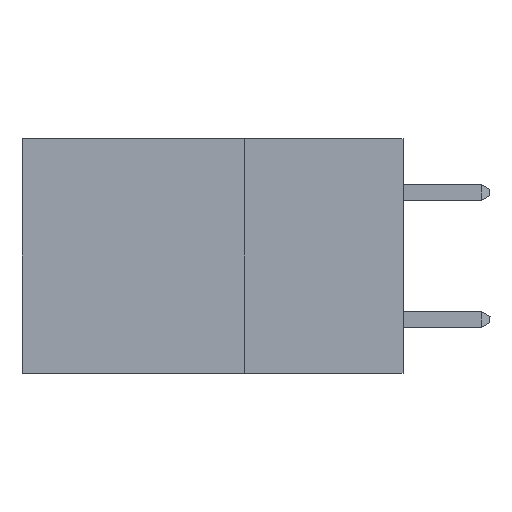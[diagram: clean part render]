
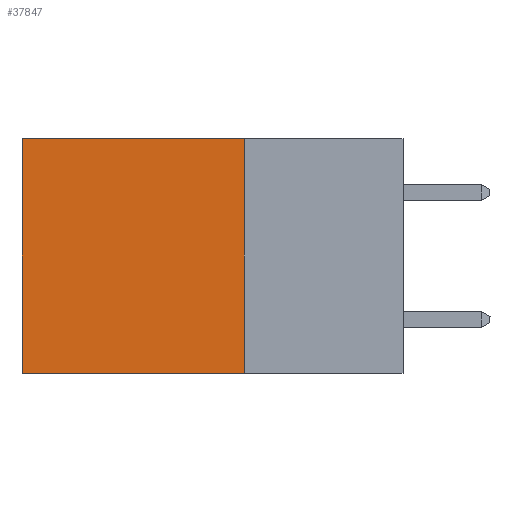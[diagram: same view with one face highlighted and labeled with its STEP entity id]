
A CAD part, left-side view. The second image highlights one B-rep face of the part: STEP entity #37847.
In plain terms, the highlighted planar face has unit normal (-1, 0, 0).
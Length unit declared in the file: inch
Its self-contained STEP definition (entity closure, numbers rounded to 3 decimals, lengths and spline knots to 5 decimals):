
#885 = CARTESIAN_POINT ( 'NONE',  ( 0.2875, 0.25, 0. ) ) ;
#1662 = DIRECTION ( 'NONE',  ( 0., 0., -1. ) ) ;
#4812 = PLANE ( 'NONE',  #25223 ) ;
#5184 = CARTESIAN_POINT ( 'NONE',  ( 0.2875, 0.25, 0. ) ) ;
#6577 = CARTESIAN_POINT ( 'NONE',  ( 0.2875, 0.25, -0.37 ) ) ;
#6785 = VECTOR ( 'NONE', #1662, 39.37008 ) ;
#6862 = VERTEX_POINT ( 'NONE', #45801 ) ;
#7627 = EDGE_CURVE ( 'NONE', #10943, #46175, #34554, .T. ) ;
#8343 = CARTESIAN_POINT ( 'NONE',  ( 0.2875, 0.25, 0. ) ) ;
#10943 = VERTEX_POINT ( 'NONE', #28861 ) ;
#11965 = EDGE_CURVE ( 'NONE', #6862, #46175, #33854, .T. ) ;
#15778 = LINE ( 'NONE', #5184, #25715 ) ;
#16038 = DIRECTION ( 'NONE',  ( 0., 0., -1. ) ) ;
#16236 = VERTEX_POINT ( 'NONE', #885 ) ;
#17128 = VECTOR ( 'NONE', #34318, 39.37008 ) ;
#18551 = VECTOR ( 'NONE', #16038, 39.37008 ) ;
#18856 = ORIENTED_EDGE ( 'NONE', *, *, #11965, .T. ) ;
#19584 = CARTESIAN_POINT ( 'NONE',  ( 0.2875, 0.6, -0.37 ) ) ;
#19651 = FACE_OUTER_BOUND ( 'NONE', #20951, .T. ) ;
#20951 = EDGE_LOOP ( 'NONE', ( #18856, #37924, #23394, #32999 ) ) ;
#23394 = ORIENTED_EDGE ( 'NONE', *, *, #41701, .F. ) ;
#25223 = AXIS2_PLACEMENT_3D ( 'NONE', #8343, #30203, #37019 ) ;
#25715 = VECTOR ( 'NONE', #37389, 39.37008 ) ;
#27074 = CARTESIAN_POINT ( 'NONE',  ( 0.2875, 0.6, 0. ) ) ;
#28861 = CARTESIAN_POINT ( 'NONE',  ( 0.2875, 0.25, -0.37 ) ) ;
#30203 = DIRECTION ( 'NONE',  ( 1., 0., 0. ) ) ;
#32070 = EDGE_CURVE ( 'NONE', #16236, #6862, #15778, .T. ) ;
#32999 = ORIENTED_EDGE ( 'NONE', *, *, #32070, .T. ) ;
#33854 = LINE ( 'NONE', #27074, #6785 ) ;
#33877 = CARTESIAN_POINT ( 'NONE',  ( 0.2875, 0.25, 0. ) ) ;
#34318 = DIRECTION ( 'NONE',  ( 0., 1., 0. ) ) ;
#34554 = LINE ( 'NONE', #6577, #17128 ) ;
#37019 = DIRECTION ( 'NONE',  ( 0., 0., -1. ) ) ;
#37389 = DIRECTION ( 'NONE',  ( 0., 1., 0. ) ) ;
#37847 = ADVANCED_FACE ( 'NONE', ( #19651 ), #4812, .F. ) ;
#37924 = ORIENTED_EDGE ( 'NONE', *, *, #7627, .F. ) ;
#40483 = LINE ( 'NONE', #33877, #18551 ) ;
#41701 = EDGE_CURVE ( 'NONE', #16236, #10943, #40483, .T. ) ;
#45801 = CARTESIAN_POINT ( 'NONE',  ( 0.2875, 0.6, 0. ) ) ;
#46175 = VERTEX_POINT ( 'NONE', #19584 ) ;
